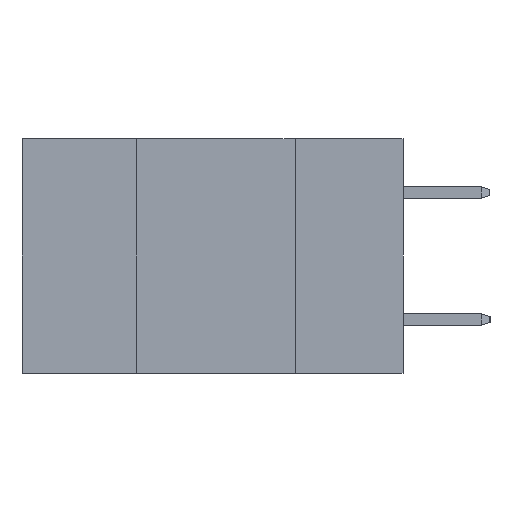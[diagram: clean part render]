
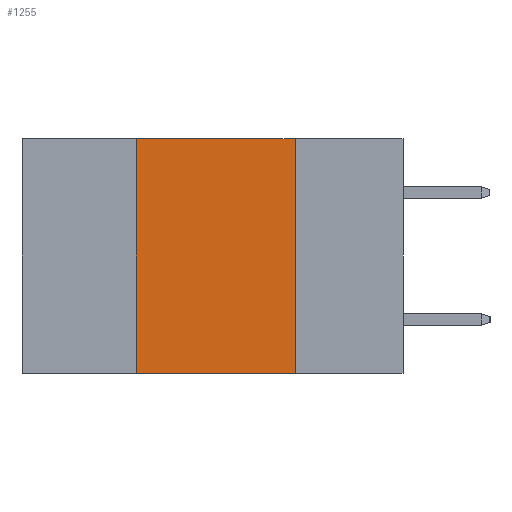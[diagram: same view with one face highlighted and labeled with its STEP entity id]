
A CAD part, left-side view. The second image highlights one B-rep face of the part: STEP entity #1255.
In plain terms, the highlighted planar face has unit normal (-1, 0, 0).
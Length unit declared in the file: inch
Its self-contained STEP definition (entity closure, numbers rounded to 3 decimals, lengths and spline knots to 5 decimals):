
#1255 = ADVANCED_FACE ( 'NONE', ( #8746 ), #16561, .F. ) ;
#1327 = VECTOR ( 'NONE', #14789, 39.37008 ) ;
#1378 = CARTESIAN_POINT ( 'NONE',  ( 0., 0.17, 0. ) ) ;
#1864 = DIRECTION ( 'NONE',  ( 0., -1., 0. ) ) ;
#2036 = VECTOR ( 'NONE', #1864, 39.37008 ) ;
#2510 = VERTEX_POINT ( 'NONE', #8086 ) ;
#2565 = ORIENTED_EDGE ( 'NONE', *, *, #13205, .T. ) ;
#2595 = CARTESIAN_POINT ( 'NONE',  ( 0., 0.17, -0.37 ) ) ;
#3021 = CARTESIAN_POINT ( 'NONE',  ( 0., 0.6, 0. ) ) ;
#3672 = DIRECTION ( 'NONE',  ( 0., 0., -1. ) ) ;
#5185 = LINE ( 'NONE', #14003, #2036 ) ;
#5535 = VERTEX_POINT ( 'NONE', #1378 ) ;
#6621 = CARTESIAN_POINT ( 'NONE',  ( 0., 0.17, 0. ) ) ;
#7455 = DIRECTION ( 'NONE',  ( 0., 0., -1. ) ) ;
#7488 = CARTESIAN_POINT ( 'NONE',  ( 0., 0.42, 0. ) ) ;
#8000 = LINE ( 'NONE', #6621, #18518 ) ;
#8086 = CARTESIAN_POINT ( 'NONE',  ( 0., 0.42, -0.37 ) ) ;
#8244 = LINE ( 'NONE', #17370, #8635 ) ;
#8635 = VECTOR ( 'NONE', #12800, 39.37008 ) ;
#8746 = FACE_OUTER_BOUND ( 'NONE', #12010, .T. ) ;
#11050 = EDGE_CURVE ( 'NONE', #5535, #15033, #8000, .T. ) ;
#11629 = CARTESIAN_POINT ( 'NONE',  ( 0., 0.42, 0. ) ) ;
#12010 = EDGE_LOOP ( 'NONE', ( #17802, #16169, #14959, #2565 ) ) ;
#12135 = AXIS2_PLACEMENT_3D ( 'NONE', #3021, #16372, #7455 ) ;
#12800 = DIRECTION ( 'NONE',  ( 0., -1., 0. ) ) ;
#13183 = EDGE_CURVE ( 'NONE', #16903, #5535, #5185, .T. ) ;
#13205 = EDGE_CURVE ( 'NONE', #2510, #15033, #8244, .T. ) ;
#14003 = CARTESIAN_POINT ( 'NONE',  ( 0., 0.6, 0. ) ) ;
#14789 = DIRECTION ( 'NONE',  ( 0., 0., 1. ) ) ;
#14959 = ORIENTED_EDGE ( 'NONE', *, *, #18385, .F. ) ;
#15033 = VERTEX_POINT ( 'NONE', #2595 ) ;
#16169 = ORIENTED_EDGE ( 'NONE', *, *, #13183, .F. ) ;
#16372 = DIRECTION ( 'NONE',  ( 1., 0., 0. ) ) ;
#16561 = PLANE ( 'NONE',  #12135 ) ;
#16903 = VERTEX_POINT ( 'NONE', #7488 ) ;
#17370 = CARTESIAN_POINT ( 'NONE',  ( 0., 0.6, -0.37 ) ) ;
#17802 = ORIENTED_EDGE ( 'NONE', *, *, #11050, .F. ) ;
#18385 = EDGE_CURVE ( 'NONE', #2510, #16903, #19255, .T. ) ;
#18518 = VECTOR ( 'NONE', #3672, 39.37008 ) ;
#19255 = LINE ( 'NONE', #11629, #1327 ) ;
